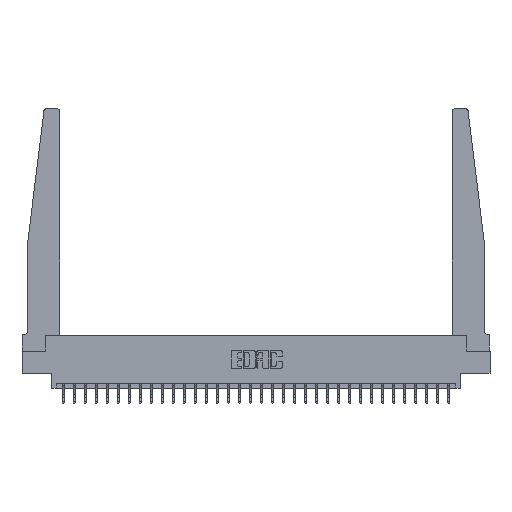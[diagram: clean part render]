
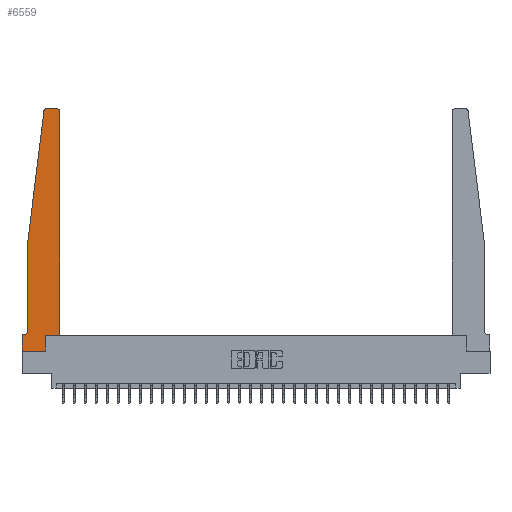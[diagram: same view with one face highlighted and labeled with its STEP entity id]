
A CAD part, top view. The second image highlights one B-rep face of the part: STEP entity #6559.
In plain terms, the highlighted planar face has unit normal (0, 0, 1).
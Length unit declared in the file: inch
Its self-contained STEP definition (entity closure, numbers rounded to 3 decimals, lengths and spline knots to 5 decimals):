
#308 = CIRCLE ( 'NONE', #18161, 0.03 ) ;
#325 = VECTOR ( 'NONE', #21788, 39.37008 ) ;
#327 = DIRECTION ( 'NONE',  ( -0.122, -0.992, 0. ) ) ;
#903 = DIRECTION ( 'NONE',  ( 0., -1., 0. ) ) ;
#1035 = LINE ( 'NONE', #5633, #3452 ) ;
#1199 = CARTESIAN_POINT ( 'NONE',  ( 0.425, 0.18, 0.37 ) ) ;
#1337 = EDGE_CURVE ( 'NONE', #15830, #17577, #13538, .T. ) ;
#2562 = VERTEX_POINT ( 'NONE', #9464 ) ;
#2846 = VERTEX_POINT ( 'NONE', #3900 ) ;
#2957 = VECTOR ( 'NONE', #8806, 39.37008 ) ;
#3304 = CARTESIAN_POINT ( 'NONE',  ( 0.015, 0.1875, 0.37 ) ) ;
#3452 = VECTOR ( 'NONE', #903, 39.37008 ) ;
#3712 = CARTESIAN_POINT ( 'NONE',  ( 0., 0., 0.37 ) ) ;
#3900 = CARTESIAN_POINT ( 'NONE',  ( 0.425, 0.18, 0.37 ) ) ;
#4672 = ORIENTED_EDGE ( 'NONE', *, *, #1337, .T. ) ;
#4876 = CARTESIAN_POINT ( 'NONE',  ( 0.065, 1.25, 0.37 ) ) ;
#5633 = CARTESIAN_POINT ( 'NONE',  ( 0., 0., 0.37 ) ) ;
#5770 = DIRECTION ( 'NONE',  ( 0., 1., 0. ) ) ;
#5944 = VERTEX_POINT ( 'NONE', #10787 ) ;
#6459 = EDGE_CURVE ( 'NONE', #29749, #18346, #6640, .T. ) ;
#6525 = AXIS2_PLACEMENT_3D ( 'NONE', #17377, #22330, #26579 ) ;
#6559 = ADVANCED_FACE ( 'NONE', ( #17936 ), #8288, .T. ) ;
#6640 = LINE ( 'NONE', #3712, #21189 ) ;
#8288 = PLANE ( 'NONE',  #20416 ) ;
#8306 = CARTESIAN_POINT ( 'NONE',  ( 0.2605, 0.18, 0.37 ) ) ;
#8700 = ORIENTED_EDGE ( 'NONE', *, *, #18327, .T. ) ;
#8806 = DIRECTION ( 'NONE',  ( 1., 0., 0. ) ) ;
#8968 = CIRCLE ( 'NONE', #6525, 0.03 ) ;
#9464 = CARTESIAN_POINT ( 'NONE',  ( 0.24675, 2.72367, 0.37 ) ) ;
#9918 = VECTOR ( 'NONE', #5770, 39.37008 ) ;
#10124 = EDGE_CURVE ( 'NONE', #14708, #29749, #1035, .T. ) ;
#10176 = VERTEX_POINT ( 'NONE', #3304 ) ;
#10683 = VERTEX_POINT ( 'NONE', #23030 ) ;
#10787 = CARTESIAN_POINT ( 'NONE',  ( 0.2605, 0.18, 0.37 ) ) ;
#11002 = LINE ( 'NONE', #8306, #19624 ) ;
#11158 = ORIENTED_EDGE ( 'NONE', *, *, #10124, .T. ) ;
#11973 = ORIENTED_EDGE ( 'NONE', *, *, #22215, .T. ) ;
#12239 = ORIENTED_EDGE ( 'NONE', *, *, #21638, .T. ) ;
#13105 = VECTOR ( 'NONE', #28190, 39.37008 ) ;
#13208 = VECTOR ( 'NONE', #327, 39.37008 ) ;
#13213 = DIRECTION ( 'NONE',  ( 0., 0., -1. ) ) ;
#13538 = LINE ( 'NONE', #18253, #20062 ) ;
#14104 = EDGE_CURVE ( 'NONE', #17577, #2562, #8968, .T. ) ;
#14175 = CARTESIAN_POINT ( 'NONE',  ( 0., 0.1875, 0.37 ) ) ;
#14258 = DIRECTION ( 'NONE',  ( 1., 0., 0. ) ) ;
#14662 = AXIS2_PLACEMENT_3D ( 'NONE', #16088, #13213, #27716 ) ;
#14708 = VERTEX_POINT ( 'NONE', #14175 ) ;
#15104 = EDGE_CURVE ( 'NONE', #5944, #2846, #20244, .T. ) ;
#15595 = CARTESIAN_POINT ( 'NONE',  ( 0.2605, 0., 0.37 ) ) ;
#15732 = CARTESIAN_POINT ( 'NONE',  ( 0.425, 0.18, 0.37 ) ) ;
#15830 = VERTEX_POINT ( 'NONE', #17343 ) ;
#15962 = DIRECTION ( 'NONE',  ( -1., 0., 0. ) ) ;
#16088 = CARTESIAN_POINT ( 'NONE',  ( 0.015, 0.2375, 0.37 ) ) ;
#16531 = DIRECTION ( 'NONE',  ( 0., 0., 1. ) ) ;
#16818 = ORIENTED_EDGE ( 'NONE', *, *, #6459, .T. ) ;
#17031 = CARTESIAN_POINT ( 'NONE',  ( 0., 0., 0.37 ) ) ;
#17343 = CARTESIAN_POINT ( 'NONE',  ( 0.395, 2.75, 0.37 ) ) ;
#17377 = CARTESIAN_POINT ( 'NONE',  ( 0.27653, 2.72, 0.37 ) ) ;
#17577 = VERTEX_POINT ( 'NONE', #19452 ) ;
#17936 = FACE_OUTER_BOUND ( 'NONE', #25004, .T. ) ;
#18018 = ORIENTED_EDGE ( 'NONE', *, *, #21029, .T. ) ;
#18110 = CARTESIAN_POINT ( 'NONE',  ( 0., 0.1875, 0.37 ) ) ;
#18161 = AXIS2_PLACEMENT_3D ( 'NONE', #28015, #16531, #14258 ) ;
#18253 = CARTESIAN_POINT ( 'NONE',  ( 0.25, 2.75, 0.37 ) ) ;
#18327 = EDGE_CURVE ( 'NONE', #2846, #10683, #21810, .T. ) ;
#18346 = VERTEX_POINT ( 'NONE', #15595 ) ;
#19452 = CARTESIAN_POINT ( 'NONE',  ( 0.27653, 2.75, 0.37 ) ) ;
#19624 = VECTOR ( 'NONE', #26869, 39.37008 ) ;
#20062 = VECTOR ( 'NONE', #15962, 39.37008 ) ;
#20244 = LINE ( 'NONE', #15732, #2957 ) ;
#20347 = CARTESIAN_POINT ( 'NONE',  ( 0.065, 0.1875, 0.37 ) ) ;
#20416 = AXIS2_PLACEMENT_3D ( 'NONE', #18110, #27299, #25023 ) ;
#20531 = CARTESIAN_POINT ( 'NONE',  ( 0.065, 1.25, 0.37 ) ) ;
#21029 = EDGE_CURVE ( 'NONE', #10683, #15830, #308, .T. ) ;
#21189 = VECTOR ( 'NONE', #29738, 39.37008 ) ;
#21638 = EDGE_CURVE ( 'NONE', #25754, #21960, #24752, .T. ) ;
#21718 = CARTESIAN_POINT ( 'NONE',  ( 0.065, 1.25, 0.37 ) ) ;
#21788 = DIRECTION ( 'NONE',  ( -1., 0., 0. ) ) ;
#21810 = LINE ( 'NONE', #1199, #9918 ) ;
#21880 = ORIENTED_EDGE ( 'NONE', *, *, #15104, .T. ) ;
#21960 = VERTEX_POINT ( 'NONE', #25283 ) ;
#22001 = EDGE_CURVE ( 'NONE', #21960, #10176, #28075, .T. ) ;
#22215 = EDGE_CURVE ( 'NONE', #2562, #25754, #25584, .T. ) ;
#22330 = DIRECTION ( 'NONE',  ( 0., 0., 1. ) ) ;
#23030 = CARTESIAN_POINT ( 'NONE',  ( 0.425, 2.72, 0.37 ) ) ;
#23649 = ORIENTED_EDGE ( 'NONE', *, *, #22001, .T. ) ;
#24033 = LINE ( 'NONE', #20347, #325 ) ;
#24161 = ORIENTED_EDGE ( 'NONE', *, *, #29401, .T. ) ;
#24752 = LINE ( 'NONE', #20531, #13105 ) ;
#25004 = EDGE_LOOP ( 'NONE', ( #4672, #26222, #11973, #12239, #23649, #25570, #11158, #16818, #24161, #21880, #8700, #18018 ) ) ;
#25023 = DIRECTION ( 'NONE',  ( 1., 0., 0. ) ) ;
#25283 = CARTESIAN_POINT ( 'NONE',  ( 0.065, 0.2375, 0.37 ) ) ;
#25570 = ORIENTED_EDGE ( 'NONE', *, *, #26870, .T. ) ;
#25584 = LINE ( 'NONE', #4876, #13208 ) ;
#25754 = VERTEX_POINT ( 'NONE', #21718 ) ;
#26222 = ORIENTED_EDGE ( 'NONE', *, *, #14104, .T. ) ;
#26579 = DIRECTION ( 'NONE',  ( 1., 0., 0. ) ) ;
#26869 = DIRECTION ( 'NONE',  ( 0., 1., 0. ) ) ;
#26870 = EDGE_CURVE ( 'NONE', #10176, #14708, #24033, .T. ) ;
#27299 = DIRECTION ( 'NONE',  ( 0., 0., 1. ) ) ;
#27716 = DIRECTION ( 'NONE',  ( -1., 0., 0. ) ) ;
#28015 = CARTESIAN_POINT ( 'NONE',  ( 0.395, 2.72, 0.37 ) ) ;
#28075 = CIRCLE ( 'NONE', #14662, 0.05 ) ;
#28190 = DIRECTION ( 'NONE',  ( 0., -1., 0. ) ) ;
#29401 = EDGE_CURVE ( 'NONE', #18346, #5944, #11002, .T. ) ;
#29738 = DIRECTION ( 'NONE',  ( 1., 0., 0. ) ) ;
#29749 = VERTEX_POINT ( 'NONE', #17031 ) ;
